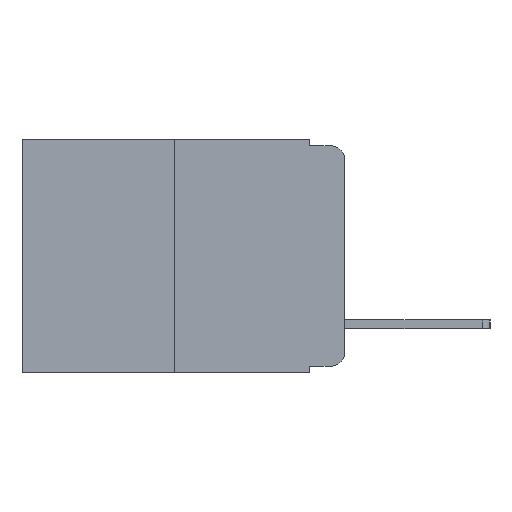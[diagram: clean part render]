
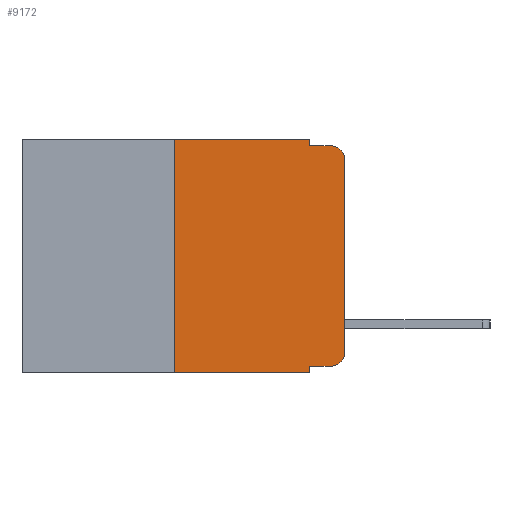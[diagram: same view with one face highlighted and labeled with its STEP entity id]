
A CAD part, left-side view. The second image highlights one B-rep face of the part: STEP entity #9172.
In plain terms, the highlighted planar face has unit normal (-1, 0, 0).
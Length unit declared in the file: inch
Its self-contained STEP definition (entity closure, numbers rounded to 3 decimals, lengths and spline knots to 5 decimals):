
#824 = EDGE_CURVE ( 'NONE', #15520, #11168, #3389, .T. ) ;
#1145 = CARTESIAN_POINT ( 'NONE',  ( 0., 0.02, -0.313 ) ) ;
#1186 = EDGE_CURVE ( 'NONE', #11833, #10924, #13599, .T. ) ;
#1327 = EDGE_CURVE ( 'NONE', #11168, #5770, #7930, .T. ) ;
#2158 = CARTESIAN_POINT ( 'NONE',  ( 0., 0.051, -0.333 ) ) ;
#2180 = LINE ( 'NONE', #13572, #12157 ) ;
#2192 = DIRECTION ( 'NONE',  ( 1., 0., 0. ) ) ;
#2328 = ORIENTED_EDGE ( 'NONE', *, *, #1186, .F. ) ;
#2472 = EDGE_CURVE ( 'NONE', #13780, #5770, #13369, .T. ) ;
#2525 = DIRECTION ( 'NONE',  ( 0., 0., -1. ) ) ;
#2575 = VECTOR ( 'NONE', #16199, 39.37008 ) ;
#3067 = DIRECTION ( 'NONE',  ( 0., 0., 1. ) ) ;
#3158 = VERTEX_POINT ( 'NONE', #14918 ) ;
#3389 = LINE ( 'NONE', #9363, #16503 ) ;
#3563 = ORIENTED_EDGE ( 'NONE', *, *, #5098, .T. ) ;
#3575 = CARTESIAN_POINT ( 'NONE',  ( 0., 0.02, -0.01 ) ) ;
#3997 = ORIENTED_EDGE ( 'NONE', *, *, #10671, .T. ) ;
#4277 = EDGE_LOOP ( 'NONE', ( #13982, #4604, #8124, #8518, #15531, #2328, #6263, #9728, #3563, #3997 ) ) ;
#4410 = VECTOR ( 'NONE', #9016, 39.37008 ) ;
#4590 = CARTESIAN_POINT ( 'NONE',  ( 0., 0.051, -0.01 ) ) ;
#4604 = ORIENTED_EDGE ( 'NONE', *, *, #2472, .T. ) ;
#4664 = EDGE_CURVE ( 'NONE', #11833, #9171, #11038, .T. ) ;
#4781 = CARTESIAN_POINT ( 'NONE',  ( 0., 0.051, -0.343 ) ) ;
#4963 = CARTESIAN_POINT ( 'NONE',  ( 0., 0., 0. ) ) ;
#5098 = EDGE_CURVE ( 'NONE', #5455, #7002, #13874, .T. ) ;
#5241 = CARTESIAN_POINT ( 'NONE',  ( 0., 0.051, -0.01 ) ) ;
#5455 = VERTEX_POINT ( 'NONE', #2158 ) ;
#5714 = CARTESIAN_POINT ( 'NONE',  ( 0., 0.25, 0. ) ) ;
#5770 = VERTEX_POINT ( 'NONE', #3575 ) ;
#5859 = CARTESIAN_POINT ( 'NONE',  ( 0., 0.473, -0.343 ) ) ;
#5883 = DIRECTION ( 'NONE',  ( 0., -1., 0. ) ) ;
#5916 = DIRECTION ( 'NONE',  ( 0., 0., -1. ) ) ;
#6263 = ORIENTED_EDGE ( 'NONE', *, *, #4664, .T. ) ;
#6435 = CARTESIAN_POINT ( 'NONE',  ( 0., 0.02, -0.333 ) ) ;
#6960 = CARTESIAN_POINT ( 'NONE',  ( 0., 0.051, -0.333 ) ) ;
#7002 = VERTEX_POINT ( 'NONE', #6435 ) ;
#7263 = DIRECTION ( 'NONE',  ( -1., 0., 0. ) ) ;
#7470 = CARTESIAN_POINT ( 'NONE',  ( 0., 0.473, 0. ) ) ;
#7479 = CARTESIAN_POINT ( 'NONE',  ( 0., 0.473, 0. ) ) ;
#7551 = DIRECTION ( 'NONE',  ( 0., -1., 0. ) ) ;
#7930 = LINE ( 'NONE', #5241, #4410 ) ;
#8124 = ORIENTED_EDGE ( 'NONE', *, *, #1327, .F. ) ;
#8518 = ORIENTED_EDGE ( 'NONE', *, *, #824, .F. ) ;
#8663 = DIRECTION ( 'NONE',  ( 0., 0., -1. ) ) ;
#9016 = DIRECTION ( 'NONE',  ( 0., -1., 0. ) ) ;
#9171 = VERTEX_POINT ( 'NONE', #4781 ) ;
#9172 = ADVANCED_FACE ( 'NONE', ( #13136 ), #10066, .F. ) ;
#9188 = CIRCLE ( 'NONE', #12746, 0.02 ) ;
#9236 = EDGE_CURVE ( 'NONE', #3158, #13780, #12369, .T. ) ;
#9363 = CARTESIAN_POINT ( 'NONE',  ( 0., 0.051, 0. ) ) ;
#9728 = ORIENTED_EDGE ( 'NONE', *, *, #11205, .F. ) ;
#10066 = PLANE ( 'NONE',  #11514 ) ;
#10382 = DIRECTION ( 'NONE',  ( -1., 0., 0. ) ) ;
#10620 = VECTOR ( 'NONE', #7551, 39.37008 ) ;
#10671 = EDGE_CURVE ( 'NONE', #7002, #3158, #9188, .T. ) ;
#10761 = CARTESIAN_POINT ( 'NONE',  ( 0., 0.25, 0. ) ) ;
#10924 = VERTEX_POINT ( 'NONE', #10761 ) ;
#11038 = LINE ( 'NONE', #5859, #14286 ) ;
#11139 = VECTOR ( 'NONE', #3067, 39.37008 ) ;
#11168 = VERTEX_POINT ( 'NONE', #4590 ) ;
#11205 = EDGE_CURVE ( 'NONE', #5455, #9171, #2180, .T. ) ;
#11338 = DIRECTION ( 'NONE',  ( 0., 0., -1. ) ) ;
#11514 = AXIS2_PLACEMENT_3D ( 'NONE', #7470, #2192, #11338 ) ;
#11616 = DIRECTION ( 'NONE',  ( 0., 0., -1. ) ) ;
#11833 = VERTEX_POINT ( 'NONE', #16041 ) ;
#11916 = EDGE_CURVE ( 'NONE', #10924, #15520, #16125, .T. ) ;
#12157 = VECTOR ( 'NONE', #5916, 39.37008 ) ;
#12369 = LINE ( 'NONE', #4963, #15237 ) ;
#12523 = CARTESIAN_POINT ( 'NONE',  ( 0., 0.051, 0. ) ) ;
#12746 = AXIS2_PLACEMENT_3D ( 'NONE', #1145, #10382, #2525 ) ;
#13136 = FACE_OUTER_BOUND ( 'NONE', #4277, .T. ) ;
#13369 = CIRCLE ( 'NONE', #16147, 0.02 ) ;
#13572 = CARTESIAN_POINT ( 'NONE',  ( 0., 0.051, 0. ) ) ;
#13599 = LINE ( 'NONE', #5714, #11139 ) ;
#13780 = VERTEX_POINT ( 'NONE', #16337 ) ;
#13874 = LINE ( 'NONE', #6960, #10620 ) ;
#13982 = ORIENTED_EDGE ( 'NONE', *, *, #9236, .T. ) ;
#14286 = VECTOR ( 'NONE', #5883, 39.37008 ) ;
#14918 = CARTESIAN_POINT ( 'NONE',  ( 0., 0., -0.313 ) ) ;
#15122 = DIRECTION ( 'NONE',  ( 0., 0., 1. ) ) ;
#15237 = VECTOR ( 'NONE', #15122, 39.37008 ) ;
#15520 = VERTEX_POINT ( 'NONE', #12523 ) ;
#15531 = ORIENTED_EDGE ( 'NONE', *, *, #11916, .F. ) ;
#15991 = CARTESIAN_POINT ( 'NONE',  ( 0., 0.02, -0.03 ) ) ;
#16041 = CARTESIAN_POINT ( 'NONE',  ( 0., 0.25, -0.343 ) ) ;
#16125 = LINE ( 'NONE', #7479, #2575 ) ;
#16147 = AXIS2_PLACEMENT_3D ( 'NONE', #15991, #7263, #11616 ) ;
#16199 = DIRECTION ( 'NONE',  ( 0., -1., 0. ) ) ;
#16337 = CARTESIAN_POINT ( 'NONE',  ( 0., 0., -0.03 ) ) ;
#16503 = VECTOR ( 'NONE', #8663, 39.37008 ) ;
